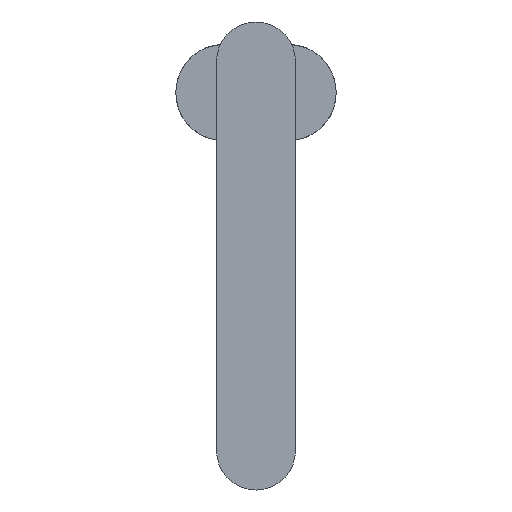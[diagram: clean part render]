
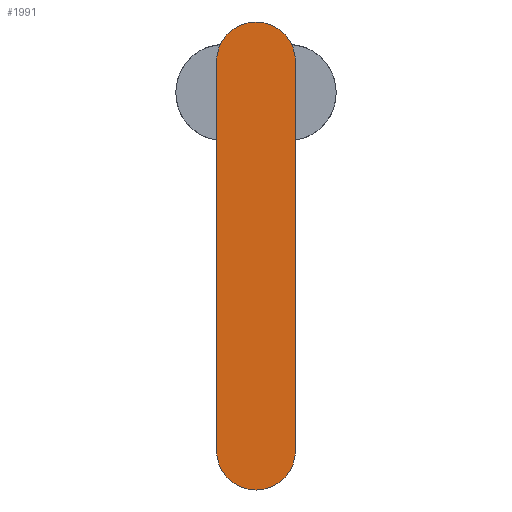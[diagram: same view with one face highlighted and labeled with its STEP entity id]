
A CAD part, left-side view. The second image highlights one B-rep face of the part: STEP entity #1991.
In plain terms, the highlighted planar face has unit normal (-1, 0, 0).
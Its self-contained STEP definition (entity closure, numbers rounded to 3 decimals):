
#55=PLANE('',#2115);
#104=FACE_OUTER_BOUND('',#208,.T.);
#208=EDGE_LOOP('',(#1471,#1472,#1473,#1474));
#291=CIRCLE('',#2109,3.124);
#293=CIRCLE('',#2114,3.124);
#540=LINE('',#9101,#630);
#554=LINE('',#10045,#644);
#630=VECTOR('',#2327,10.);
#644=VECTOR('',#2365,10.);
#769=VERTEX_POINT('',#9098);
#770=VERTEX_POINT('',#9100);
#779=VERTEX_POINT('',#10035);
#781=VERTEX_POINT('',#10043);
#1014=EDGE_CURVE('',#770,#769,#540,.T.);
#1033=EDGE_CURVE('',#779,#769,#291,.T.);
#1037=EDGE_CURVE('',#779,#781,#554,.T.);
#1038=EDGE_CURVE('',#770,#781,#293,.T.);
#1471=ORIENTED_EDGE('',*,*,#1038,.F.);
#1472=ORIENTED_EDGE('',*,*,#1014,.T.);
#1473=ORIENTED_EDGE('',*,*,#1033,.F.);
#1474=ORIENTED_EDGE('',*,*,#1037,.T.);
#1991=ADVANCED_FACE('',(#104),#55,.F.);
#2109=AXIS2_PLACEMENT_3D('',#10037,#2355,#2356);
#2114=AXIS2_PLACEMENT_3D('',#10047,#2368,#2369);
#2115=AXIS2_PLACEMENT_3D('',#10048,#2370,#2371);
#2327=DIRECTION('',(0.,0.,-1.));
#2355=DIRECTION('center_axis',(1.,0.,0.));
#2356=DIRECTION('ref_axis',(0.,0.,-1.));
#2365=DIRECTION('',(0.,0.,1.));
#2368=DIRECTION('center_axis',(1.,0.,0.));
#2369=DIRECTION('ref_axis',(0.,0.,-1.));
#2370=DIRECTION('center_axis',(1.,0.,0.));
#2371=DIRECTION('ref_axis',(0.,0.,-1.));
#9098=CARTESIAN_POINT('',(0.,3.124,-15.4));
#9100=CARTESIAN_POINT('',(0.,3.124,15.4));
#9101=CARTESIAN_POINT('',(0.,3.124,18.542));
#10035=CARTESIAN_POINT('',(0.,-3.124,-15.4));
#10037=CARTESIAN_POINT('Origin',(0.,0.,-15.4));
#10043=CARTESIAN_POINT('',(0.,-3.124,15.4));
#10045=CARTESIAN_POINT('',(0.,-3.124,-18.542));
#10047=CARTESIAN_POINT('Origin',(0.,0.,15.4));
#10048=CARTESIAN_POINT('Origin',(0.,0.,0.));
